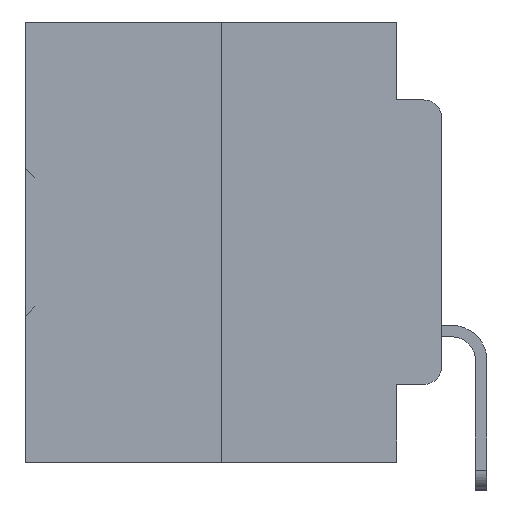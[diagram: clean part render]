
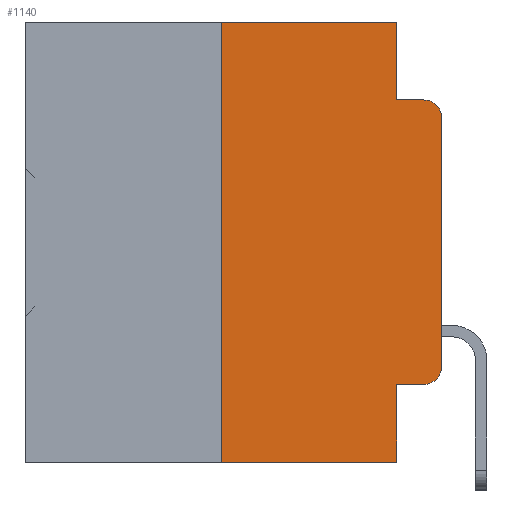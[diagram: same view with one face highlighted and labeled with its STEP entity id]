
A CAD part, left-side view. The second image highlights one B-rep face of the part: STEP entity #1140.
In plain terms, the highlighted planar face has unit normal (-1, 0, 0).
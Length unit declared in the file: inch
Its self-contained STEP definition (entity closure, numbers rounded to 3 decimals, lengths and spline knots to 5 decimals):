
#616 = EDGE_CURVE ( 'NONE', #37206, #6627, #37069, .T. ) ;
#687 = CARTESIAN_POINT ( 'NONE',  ( 0., 0.051, -0.4115 ) ) ;
#1007 = CARTESIAN_POINT ( 'NONE',  ( 0., 0.25, 0. ) ) ;
#1119 = EDGE_CURVE ( 'NONE', #5557, #27537, #27412, .T. ) ;
#1140 = ADVANCED_FACE ( 'NONE', ( #16984 ), #11868, .F. ) ;
#1745 = ORIENTED_EDGE ( 'NONE', *, *, #17811, .F. ) ;
#1972 = AXIS2_PLACEMENT_3D ( 'NONE', #38118, #20906, #2648 ) ;
#2066 = VECTOR ( 'NONE', #24755, 39.37008 ) ;
#2490 = ORIENTED_EDGE ( 'NONE', *, *, #19725, .F. ) ;
#2495 = CARTESIAN_POINT ( 'NONE',  ( 0., 0.051, -0.0885 ) ) ;
#2625 = CARTESIAN_POINT ( 'NONE',  ( 0., 0.051, -0.0885 ) ) ;
#2648 = DIRECTION ( 'NONE',  ( 0., 0., -1. ) ) ;
#3111 = LINE ( 'NONE', #30412, #2066 ) ;
#3327 = EDGE_CURVE ( 'NONE', #22680, #5557, #38305, .T. ) ;
#4573 = VERTEX_POINT ( 'NONE', #21209 ) ;
#5049 = DIRECTION ( 'NONE',  ( 0., 0., 1. ) ) ;
#5475 = CARTESIAN_POINT ( 'NONE',  ( 0., 0.473, 0. ) ) ;
#5485 = CIRCLE ( 'NONE', #1972, 0.02 ) ;
#5510 = EDGE_CURVE ( 'NONE', #22680, #20931, #36393, .T. ) ;
#5557 = VERTEX_POINT ( 'NONE', #11972 ) ;
#6024 = VECTOR ( 'NONE', #25710, 39.37008 ) ;
#6627 = VERTEX_POINT ( 'NONE', #37080 ) ;
#8644 = DIRECTION ( 'NONE',  ( 0., -1., 0. ) ) ;
#8769 = ORIENTED_EDGE ( 'NONE', *, *, #5510, .F. ) ;
#9063 = LINE ( 'NONE', #15295, #29832 ) ;
#9129 = LINE ( 'NONE', #37368, #23079 ) ;
#10383 = CARTESIAN_POINT ( 'NONE',  ( 0., 0.051, -0.5 ) ) ;
#10706 = CARTESIAN_POINT ( 'NONE',  ( 0., 0., -0.1085 ) ) ;
#11825 = AXIS2_PLACEMENT_3D ( 'NONE', #32415, #15017, #35229 ) ;
#11868 = PLANE ( 'NONE',  #23641 ) ;
#11972 = CARTESIAN_POINT ( 'NONE',  ( 0., 0.02, -0.4115 ) ) ;
#12114 = CARTESIAN_POINT ( 'NONE',  ( 0., 0.473, 0. ) ) ;
#13096 = VECTOR ( 'NONE', #8644, 39.37008 ) ;
#13458 = EDGE_CURVE ( 'NONE', #35937, #20931, #3111, .T. ) ;
#14229 = DIRECTION ( 'NONE',  ( 0., -1., 0. ) ) ;
#14297 = LINE ( 'NONE', #37025, #6024 ) ;
#15017 = DIRECTION ( 'NONE',  ( -1., 0., 0. ) ) ;
#15295 = CARTESIAN_POINT ( 'NONE',  ( 0., 0., 0. ) ) ;
#16092 = VECTOR ( 'NONE', #20883, 39.37008 ) ;
#16827 = ORIENTED_EDGE ( 'NONE', *, *, #3327, .T. ) ;
#16984 = FACE_OUTER_BOUND ( 'NONE', #19426, .T. ) ;
#17707 = CARTESIAN_POINT ( 'NONE',  ( 0., 0.051, 0. ) ) ;
#17811 = EDGE_CURVE ( 'NONE', #35937, #37206, #9129, .T. ) ;
#18104 = DIRECTION ( 'NONE',  ( 0., 0., -1. ) ) ;
#18659 = ORIENTED_EDGE ( 'NONE', *, *, #13458, .T. ) ;
#18797 = EDGE_CURVE ( 'NONE', #27537, #29374, #9063, .T. ) ;
#19426 = EDGE_LOOP ( 'NONE', ( #23387, #32889, #22019, #2490, #34475, #1745, #18659, #8769, #16827, #22003 ) ) ;
#19725 = EDGE_CURVE ( 'NONE', #6627, #19929, #14297, .T. ) ;
#19929 = VERTEX_POINT ( 'NONE', #2495 ) ;
#20883 = DIRECTION ( 'NONE',  ( 0., -1., 0. ) ) ;
#20906 = DIRECTION ( 'NONE',  ( -1., 0., 0. ) ) ;
#20931 = VERTEX_POINT ( 'NONE', #10383 ) ;
#21094 = DIRECTION ( 'NONE',  ( 0., 0., 1. ) ) ;
#21209 = CARTESIAN_POINT ( 'NONE',  ( 0., 0.02, -0.0885 ) ) ;
#21640 = EDGE_CURVE ( 'NONE', #19929, #4573, #31525, .T. ) ;
#21975 = VECTOR ( 'NONE', #29271, 39.37008 ) ;
#22003 = ORIENTED_EDGE ( 'NONE', *, *, #1119, .T. ) ;
#22019 = ORIENTED_EDGE ( 'NONE', *, *, #21640, .F. ) ;
#22680 = VERTEX_POINT ( 'NONE', #687 ) ;
#23079 = VECTOR ( 'NONE', #5049, 39.37008 ) ;
#23387 = ORIENTED_EDGE ( 'NONE', *, *, #18797, .T. ) ;
#23641 = AXIS2_PLACEMENT_3D ( 'NONE', #12114, #35340, #18104 ) ;
#24755 = DIRECTION ( 'NONE',  ( 0., -1., 0. ) ) ;
#25710 = DIRECTION ( 'NONE',  ( 0., 0., -1. ) ) ;
#25831 = CARTESIAN_POINT ( 'NONE',  ( 0., 0.051, -0.4115 ) ) ;
#27412 = CIRCLE ( 'NONE', #11825, 0.02 ) ;
#27537 = VERTEX_POINT ( 'NONE', #28669 ) ;
#28669 = CARTESIAN_POINT ( 'NONE',  ( 0., 0., -0.3915 ) ) ;
#29271 = DIRECTION ( 'NONE',  ( 0., 0., -1. ) ) ;
#29374 = VERTEX_POINT ( 'NONE', #10706 ) ;
#29832 = VECTOR ( 'NONE', #21094, 39.37008 ) ;
#30412 = CARTESIAN_POINT ( 'NONE',  ( 0., 0.473, -0.5 ) ) ;
#30822 = VECTOR ( 'NONE', #14229, 39.37008 ) ;
#31394 = EDGE_CURVE ( 'NONE', #29374, #4573, #5485, .T. ) ;
#31525 = LINE ( 'NONE', #2625, #16092 ) ;
#31747 = CARTESIAN_POINT ( 'NONE',  ( 0., 0.25, -0.5 ) ) ;
#32415 = CARTESIAN_POINT ( 'NONE',  ( 0., 0.02, -0.3915 ) ) ;
#32889 = ORIENTED_EDGE ( 'NONE', *, *, #31394, .T. ) ;
#34475 = ORIENTED_EDGE ( 'NONE', *, *, #616, .F. ) ;
#35229 = DIRECTION ( 'NONE',  ( 0., 0., -1. ) ) ;
#35340 = DIRECTION ( 'NONE',  ( 1., 0., 0. ) ) ;
#35937 = VERTEX_POINT ( 'NONE', #31747 ) ;
#36393 = LINE ( 'NONE', #17707, #21975 ) ;
#37025 = CARTESIAN_POINT ( 'NONE',  ( 0., 0.051, 0. ) ) ;
#37069 = LINE ( 'NONE', #5475, #13096 ) ;
#37080 = CARTESIAN_POINT ( 'NONE',  ( 0., 0.051, 0. ) ) ;
#37206 = VERTEX_POINT ( 'NONE', #1007 ) ;
#37368 = CARTESIAN_POINT ( 'NONE',  ( 0., 0.25, 0. ) ) ;
#38118 = CARTESIAN_POINT ( 'NONE',  ( 0., 0.02, -0.1085 ) ) ;
#38305 = LINE ( 'NONE', #25831, #30822 ) ;
